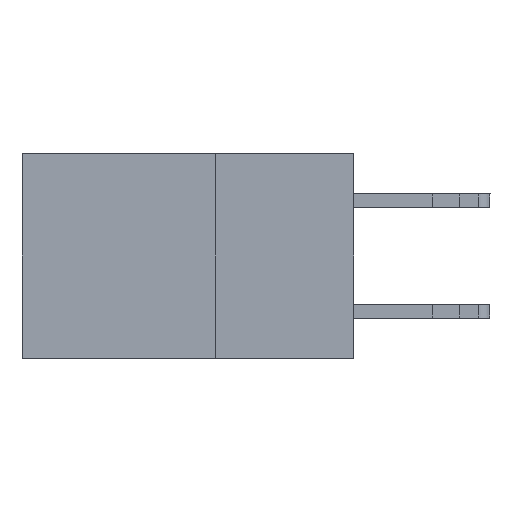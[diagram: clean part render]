
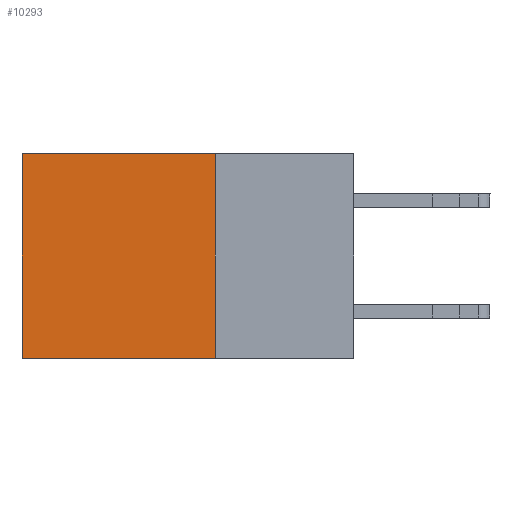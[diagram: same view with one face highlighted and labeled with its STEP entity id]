
A CAD part, left-side view. The second image highlights one B-rep face of the part: STEP entity #10293.
In plain terms, the highlighted planar face has unit normal (-1, 0, 0).
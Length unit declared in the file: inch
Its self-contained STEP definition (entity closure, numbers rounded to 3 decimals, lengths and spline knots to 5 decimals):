
#2855 = EDGE_CURVE ( 'NONE', #18518, #19465, #32407, .T. ) ;
#3771 = VECTOR ( 'NONE', #11723, 39.37008 ) ;
#5966 = VECTOR ( 'NONE', #9615, 39.37008 ) ;
#6404 = CARTESIAN_POINT ( 'NONE',  ( 0.2875, 0.25, 0. ) ) ;
#6613 = EDGE_CURVE ( 'NONE', #13624, #19465, #11174, .T. ) ;
#7537 = CARTESIAN_POINT ( 'NONE',  ( 0.2875, 0.25, 0. ) ) ;
#8761 = AXIS2_PLACEMENT_3D ( 'NONE', #6404, #8950, #31144 ) ;
#8950 = DIRECTION ( 'NONE',  ( 1., 0., 0. ) ) ;
#8966 = CARTESIAN_POINT ( 'NONE',  ( 0.2875, 0.6, 0. ) ) ;
#9615 = DIRECTION ( 'NONE',  ( 0., 1., 0. ) ) ;
#9688 = EDGE_LOOP ( 'NONE', ( #31424, #23714, #13911, #17276 ) ) ;
#10293 = ADVANCED_FACE ( 'NONE', ( #26922 ), #34086, .F. ) ;
#11174 = LINE ( 'NONE', #8966, #3771 ) ;
#11571 = CARTESIAN_POINT ( 'NONE',  ( 0.2875, 0.6, 0. ) ) ;
#11680 = VECTOR ( 'NONE', #21325, 39.37008 ) ;
#11723 = DIRECTION ( 'NONE',  ( 0., 0., -1. ) ) ;
#12244 = CARTESIAN_POINT ( 'NONE',  ( 0.2875, 0.25, -0.37 ) ) ;
#12451 = CARTESIAN_POINT ( 'NONE',  ( 0.2875, 0.6, -0.37 ) ) ;
#13624 = VERTEX_POINT ( 'NONE', #11571 ) ;
#13911 = ORIENTED_EDGE ( 'NONE', *, *, #34174, .F. ) ;
#14590 = CARTESIAN_POINT ( 'NONE',  ( 0.2875, 0.25, 0. ) ) ;
#15860 = VECTOR ( 'NONE', #24463, 39.37008 ) ;
#17276 = ORIENTED_EDGE ( 'NONE', *, *, #32220, .T. ) ;
#18518 = VERTEX_POINT ( 'NONE', #21844 ) ;
#19465 = VERTEX_POINT ( 'NONE', #12451 ) ;
#21325 = DIRECTION ( 'NONE',  ( 0., 1., 0. ) ) ;
#21780 = CARTESIAN_POINT ( 'NONE',  ( 0.2875, 0.25, 0. ) ) ;
#21844 = CARTESIAN_POINT ( 'NONE',  ( 0.2875, 0.25, -0.37 ) ) ;
#23714 = ORIENTED_EDGE ( 'NONE', *, *, #2855, .F. ) ;
#23810 = LINE ( 'NONE', #7537, #11680 ) ;
#24463 = DIRECTION ( 'NONE',  ( 0., 0., -1. ) ) ;
#26112 = VERTEX_POINT ( 'NONE', #14590 ) ;
#26922 = FACE_OUTER_BOUND ( 'NONE', #9688, .T. ) ;
#28913 = LINE ( 'NONE', #21780, #15860 ) ;
#31144 = DIRECTION ( 'NONE',  ( 0., 0., -1. ) ) ;
#31424 = ORIENTED_EDGE ( 'NONE', *, *, #6613, .T. ) ;
#32220 = EDGE_CURVE ( 'NONE', #26112, #13624, #23810, .T. ) ;
#32407 = LINE ( 'NONE', #12244, #5966 ) ;
#34086 = PLANE ( 'NONE',  #8761 ) ;
#34174 = EDGE_CURVE ( 'NONE', #26112, #18518, #28913, .T. ) ;
